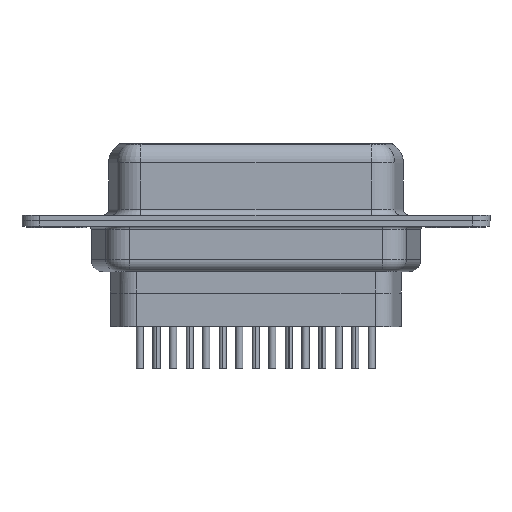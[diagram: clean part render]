
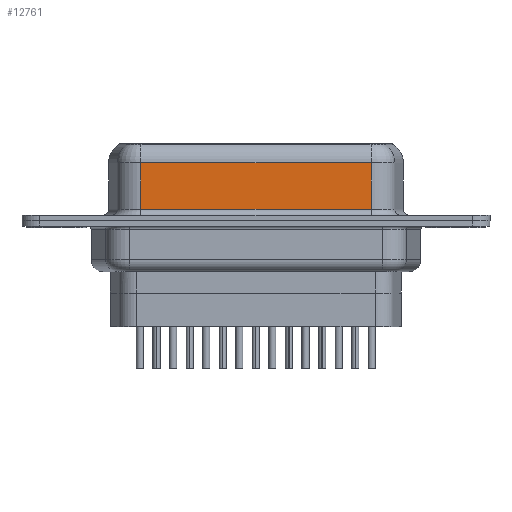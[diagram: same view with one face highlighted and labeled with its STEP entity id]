
A CAD part, front view. The second image highlights one B-rep face of the part: STEP entity #12761.
In plain terms, the highlighted planar face has unit normal (0, -1, 0).
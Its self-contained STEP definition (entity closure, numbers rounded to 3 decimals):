
#981 = DIRECTION ( 'NONE',  ( 0., 0., -1. ) ) ;
#1026 = CARTESIAN_POINT ( 'NONE',  ( 7.023, -3.95, 0.95 ) ) ;
#1158 = DIRECTION ( 'NONE',  ( -1., 0., 0. ) ) ;
#1277 = EDGE_CURVE ( 'NONE', #17454, #13447, #9820, .T. ) ;
#1523 = VECTOR ( 'NONE', #15092, 1000. ) ;
#2937 = EDGE_CURVE ( 'NONE', #17454, #19746, #13613, .T. ) ;
#3033 = FACE_OUTER_BOUND ( 'NONE', #5765, .T. ) ;
#4666 = CARTESIAN_POINT ( 'NONE',  ( 7.023, -3.95, 4.85 ) ) ;
#4743 = CARTESIAN_POINT ( 'NONE',  ( 26.297, -3.95, 6.6 ) ) ;
#5765 = EDGE_LOOP ( 'NONE', ( #20613, #21242, #11257, #9993 ) ) ;
#6725 = EDGE_CURVE ( 'NONE', #13447, #21821, #21005, .T. ) ;
#7119 = PLANE ( 'NONE',  #17697 ) ;
#7793 = CARTESIAN_POINT ( 'NONE',  ( 26.297, -3.95, 0.95 ) ) ;
#9311 = EDGE_CURVE ( 'NONE', #21821, #19746, #11268, .T. ) ;
#9820 = LINE ( 'NONE', #11829, #20934 ) ;
#9993 = ORIENTED_EDGE ( 'NONE', *, *, #9311, .T. ) ;
#10500 = DIRECTION ( 'NONE',  ( 0., 0., 1. ) ) ;
#11257 = ORIENTED_EDGE ( 'NONE', *, *, #6725, .T. ) ;
#11268 = LINE ( 'NONE', #7793, #1523 ) ;
#11829 = CARTESIAN_POINT ( 'NONE',  ( 26.297, -3.95, 4.85 ) ) ;
#12046 = DIRECTION ( 'NONE',  ( 0., 0., -1. ) ) ;
#12761 = ADVANCED_FACE ( 'NONE', ( #3033 ), #7119, .F. ) ;
#12939 = CARTESIAN_POINT ( 'NONE',  ( 26.297, -3.95, 4.85 ) ) ;
#13447 = VERTEX_POINT ( 'NONE', #4666 ) ;
#13613 = LINE ( 'NONE', #4743, #15285 ) ;
#14431 = DIRECTION ( 'NONE',  ( 0., 1., 0. ) ) ;
#15092 = DIRECTION ( 'NONE',  ( 1., 0., 0. ) ) ;
#15285 = VECTOR ( 'NONE', #12046, 1000. ) ;
#17454 = VERTEX_POINT ( 'NONE', #12939 ) ;
#17557 = VECTOR ( 'NONE', #981, 1000. ) ;
#17697 = AXIS2_PLACEMENT_3D ( 'NONE', #23418, #14431, #10500 ) ;
#19746 = VERTEX_POINT ( 'NONE', #21283 ) ;
#20613 = ORIENTED_EDGE ( 'NONE', *, *, #2937, .F. ) ;
#20934 = VECTOR ( 'NONE', #1158, 1000. ) ;
#21005 = LINE ( 'NONE', #22386, #17557 ) ;
#21242 = ORIENTED_EDGE ( 'NONE', *, *, #1277, .T. ) ;
#21283 = CARTESIAN_POINT ( 'NONE',  ( 26.297, -3.95, 0.95 ) ) ;
#21821 = VERTEX_POINT ( 'NONE', #1026 ) ;
#22386 = CARTESIAN_POINT ( 'NONE',  ( 7.023, -3.95, 6.6 ) ) ;
#23418 = CARTESIAN_POINT ( 'NONE',  ( 26.297, -3.95, 6.6 ) ) ;
